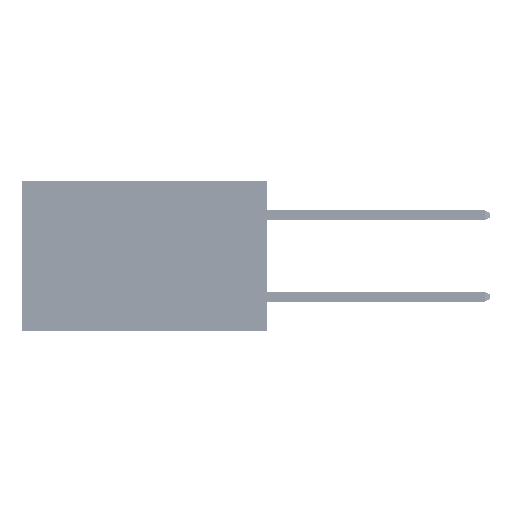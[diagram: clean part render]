
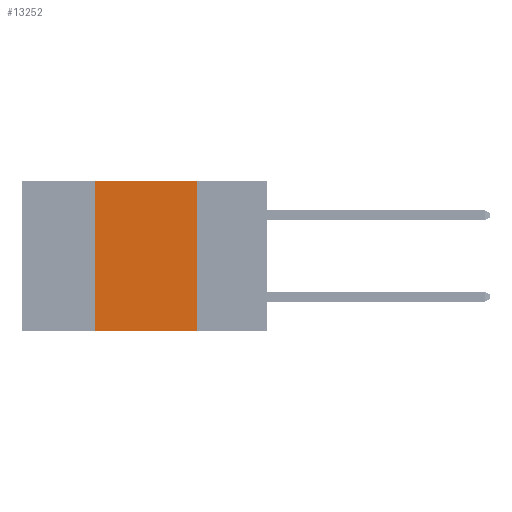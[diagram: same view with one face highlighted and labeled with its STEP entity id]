
A CAD part, left-side view. The second image highlights one B-rep face of the part: STEP entity #13252.
In plain terms, the highlighted planar face has unit normal (-1, 0, 0).
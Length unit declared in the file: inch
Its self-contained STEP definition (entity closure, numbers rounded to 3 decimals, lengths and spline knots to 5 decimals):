
#279 = PLANE ( 'NONE',  #16538 ) ;
#1845 = VECTOR ( 'NONE', #47240, 39.37008 ) ;
#3289 = DIRECTION ( 'NONE',  ( 0., 0., -1. ) ) ;
#3995 = DIRECTION ( 'NONE',  ( 0., 0., 1. ) ) ;
#5065 = EDGE_LOOP ( 'NONE', ( #32701, #40879, #17457, #10841 ) ) ;
#10841 = ORIENTED_EDGE ( 'NONE', *, *, #30027, .T. ) ;
#11265 = CARTESIAN_POINT ( 'NONE',  ( 0., 0.17, 0. ) ) ;
#12618 = DIRECTION ( 'NONE',  ( 0., -1., 0. ) ) ;
#13252 = ADVANCED_FACE ( 'NONE', ( #48171 ), #279, .F. ) ;
#15093 = DIRECTION ( 'NONE',  ( 1., 0., 0. ) ) ;
#15785 = CARTESIAN_POINT ( 'NONE',  ( 0., 0.42, 0. ) ) ;
#16538 = AXIS2_PLACEMENT_3D ( 'NONE', #22437, #15093, #26358 ) ;
#16973 = VECTOR ( 'NONE', #3289, 39.37008 ) ;
#17457 = ORIENTED_EDGE ( 'NONE', *, *, #35949, .F. ) ;
#17489 = VECTOR ( 'NONE', #12618, 39.37008 ) ;
#22437 = CARTESIAN_POINT ( 'NONE',  ( 0., 0.6, 0. ) ) ;
#26358 = DIRECTION ( 'NONE',  ( 0., 0., -1. ) ) ;
#27479 = LINE ( 'NONE', #46709, #17489 ) ;
#28749 = VERTEX_POINT ( 'NONE', #11265 ) ;
#30027 = EDGE_CURVE ( 'NONE', #42372, #46852, #33556, .T. ) ;
#30231 = CARTESIAN_POINT ( 'NONE',  ( 0., 0.42, 0. ) ) ;
#31526 = EDGE_CURVE ( 'NONE', #28749, #46852, #43360, .T. ) ;
#32701 = ORIENTED_EDGE ( 'NONE', *, *, #31526, .F. ) ;
#33161 = CARTESIAN_POINT ( 'NONE',  ( 0., 0.17, 0. ) ) ;
#33556 = LINE ( 'NONE', #39993, #1845 ) ;
#35949 = EDGE_CURVE ( 'NONE', #42372, #36368, #46330, .T. ) ;
#36368 = VERTEX_POINT ( 'NONE', #15785 ) ;
#39993 = CARTESIAN_POINT ( 'NONE',  ( 0., 0.6, -0.37 ) ) ;
#40879 = ORIENTED_EDGE ( 'NONE', *, *, #45466, .F. ) ;
#42372 = VERTEX_POINT ( 'NONE', #46808 ) ;
#43360 = LINE ( 'NONE', #33161, #16973 ) ;
#45466 = EDGE_CURVE ( 'NONE', #36368, #28749, #27479, .T. ) ;
#45490 = CARTESIAN_POINT ( 'NONE',  ( 0., 0.17, -0.37 ) ) ;
#46330 = LINE ( 'NONE', #30231, #47478 ) ;
#46709 = CARTESIAN_POINT ( 'NONE',  ( 0., 0.6, 0. ) ) ;
#46808 = CARTESIAN_POINT ( 'NONE',  ( 0., 0.42, -0.37 ) ) ;
#46852 = VERTEX_POINT ( 'NONE', #45490 ) ;
#47240 = DIRECTION ( 'NONE',  ( 0., -1., 0. ) ) ;
#47478 = VECTOR ( 'NONE', #3995, 39.37008 ) ;
#48171 = FACE_OUTER_BOUND ( 'NONE', #5065, .T. ) ;
